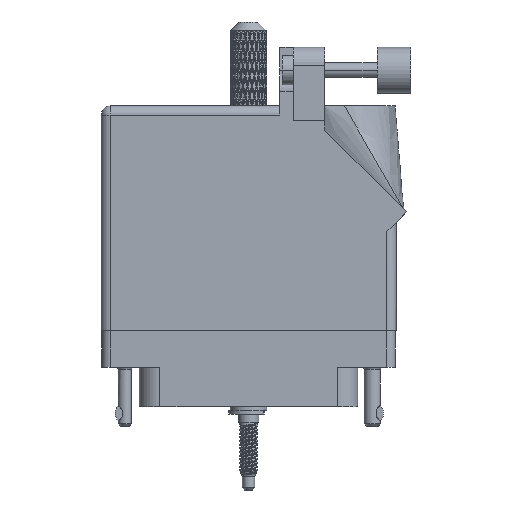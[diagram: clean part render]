
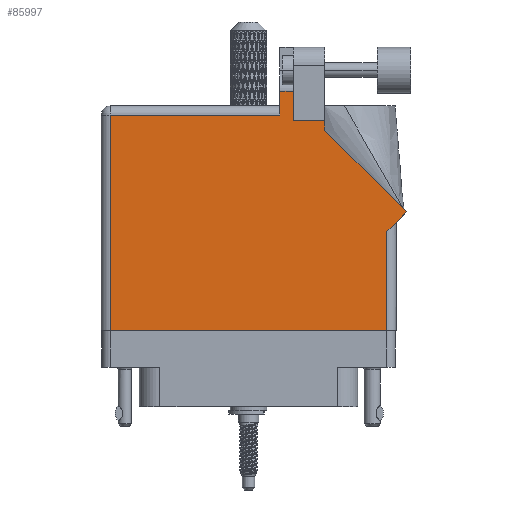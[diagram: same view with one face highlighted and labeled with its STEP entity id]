
A CAD part, front view. The second image highlights one B-rep face of the part: STEP entity #85997.
In plain terms, the highlighted face is planar.
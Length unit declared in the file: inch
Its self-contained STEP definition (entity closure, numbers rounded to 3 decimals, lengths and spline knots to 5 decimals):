
#2306 = VERTEX_POINT ( 'NONE', #101759 ) ;
#2897 = DIRECTION ( 'NONE',  ( 0., 1., 0. ) ) ;
#3239 = CARTESIAN_POINT ( 'NONE',  ( 0.212, 1.368, 0.455 ) ) ;
#4453 = DIRECTION ( 'NONE',  ( -1., 0., 0. ) ) ;
#6810 = DIRECTION ( 'NONE',  ( 0., 1., 0. ) ) ;
#7389 = VERTEX_POINT ( 'NONE', #38934 ) ;
#9613 = VERTEX_POINT ( 'NONE', #34563 ) ;
#9831 = DIRECTION ( 'NONE',  ( 0., -1., 0. ) ) ;
#12587 = ORIENTED_EDGE ( 'NONE', *, *, #70908, .T. ) ;
#12631 = VERTEX_POINT ( 'NONE', #112125 ) ;
#15644 = VECTOR ( 'NONE', #4453, 39.37008 ) ;
#15901 = CARTESIAN_POINT ( 'NONE',  ( 0.63677, 1.5315, 0.455 ) ) ;
#16752 = VECTOR ( 'NONE', #88255, 39.37008 ) ;
#16868 = FACE_OUTER_BOUND ( 'NONE', #62920, .T. ) ;
#25154 = LINE ( 'NONE', #15901, #16752 ) ;
#26247 = ORIENTED_EDGE ( 'NONE', *, *, #63996, .T. ) ;
#26473 = LINE ( 'NONE', #26677, #29269 ) ;
#26677 = CARTESIAN_POINT ( 'NONE',  ( 0.212, 1.43, 0.455 ) ) ;
#26872 = DIRECTION ( 'NONE',  ( -0.707, 0.707, 0. ) ) ;
#27418 = ORIENTED_EDGE ( 'NONE', *, *, #92689, .T. ) ;
#29269 = VECTOR ( 'NONE', #9831, 39.37008 ) ;
#30598 = ORIENTED_EDGE ( 'NONE', *, *, #83921, .T. ) ;
#31255 = ORIENTED_EDGE ( 'NONE', *, *, #103829, .T. ) ;
#32099 = CARTESIAN_POINT ( 'NONE',  ( -0.943, -0.1, 0.455 ) ) ;
#33418 = VERTEX_POINT ( 'NONE', #100658 ) ;
#34277 = CARTESIAN_POINT ( 'NONE',  ( -1.005, -0.1, 0.455 ) ) ;
#34563 = CARTESIAN_POINT ( 'NONE',  ( 0.212, 1.5315, 0.455 ) ) ;
#34659 = DIRECTION ( 'NONE',  ( 1., 0., 0. ) ) ;
#35789 = DIRECTION ( 'NONE',  ( 0., 0., -1. ) ) ;
#37146 = VECTOR ( 'NONE', #2897, 39.37008 ) ;
#38934 = CARTESIAN_POINT ( 'NONE',  ( 0.519, 1.33, 0.455 ) ) ;
#39125 = LINE ( 'NONE', #103367, #89053 ) ;
#39825 = CARTESIAN_POINT ( 'NONE',  ( 1.005, 0.637, 0.455 ) ) ;
#41065 = CARTESIAN_POINT ( 'NONE',  ( -1.005, 1.368, 0.455 ) ) ;
#43443 = CARTESIAN_POINT ( 'NONE',  ( 0.519, 1.26442, 0.455 ) ) ;
#43449 = VECTOR ( 'NONE', #89734, 39.37008 ) ;
#44180 = VECTOR ( 'NONE', #103181, 39.37008 ) ;
#44308 = PLANE ( 'NONE',  #67310 ) ;
#45299 = EDGE_CURVE ( 'NONE', #111157, #33418, #77032, .T. ) ;
#48701 = LINE ( 'NONE', #58874, #55599 ) ;
#52545 = VECTOR ( 'NONE', #111416, 39.37008 ) ;
#53640 = CARTESIAN_POINT ( 'NONE',  ( -1.005, 1.43, 0.455 ) ) ;
#55599 = VECTOR ( 'NONE', #59237, 39.37008 ) ;
#57001 = EDGE_CURVE ( 'NONE', #91630, #70174, #70779, .T. ) ;
#57333 = ORIENTED_EDGE ( 'NONE', *, *, #57001, .T. ) ;
#58874 = CARTESIAN_POINT ( 'NONE',  ( 0.519, 1.26442, 0.455 ) ) ;
#59237 = DIRECTION ( 'NONE',  ( 0., 1., 0. ) ) ;
#59428 = CARTESIAN_POINT ( 'NONE',  ( 0.306, 1.5315, 0.455 ) ) ;
#62920 = EDGE_LOOP ( 'NONE', ( #31255, #12587, #73707, #26247, #63160, #97047, #86370, #27418, #57333, #86699, #30598 ) ) ;
#63160 = ORIENTED_EDGE ( 'NONE', *, *, #91915, .T. ) ;
#63996 = EDGE_CURVE ( 'NONE', #86581, #2306, #103402, .T. ) ;
#66925 = EDGE_CURVE ( 'NONE', #70174, #7389, #48701, .T. ) ;
#67134 = LINE ( 'NONE', #114699, #43449 ) ;
#67310 = AXIS2_PLACEMENT_3D ( 'NONE', #53640, #35789, #114741 ) ;
#69325 = LINE ( 'NONE', #102088, #37146 ) ;
#70174 = VERTEX_POINT ( 'NONE', #43443 ) ;
#70779 = LINE ( 'NONE', #113625, #90266 ) ;
#70908 = EDGE_CURVE ( 'NONE', #93384, #9613, #25154, .T. ) ;
#73464 = LINE ( 'NONE', #39825, #44180 ) ;
#73707 = ORIENTED_EDGE ( 'NONE', *, *, #86479, .T. ) ;
#77032 = LINE ( 'NONE', #34277, #93613 ) ;
#83583 = VERTEX_POINT ( 'NONE', #89110 ) ;
#83921 = EDGE_CURVE ( 'NONE', #7389, #83583, #67134, .T. ) ;
#85997 = ADVANCED_FACE ( 'NONE', ( #16868 ), #44308, .F. ) ;
#86370 = ORIENTED_EDGE ( 'NONE', *, *, #92242, .T. ) ;
#86479 = EDGE_CURVE ( 'NONE', #9613, #86581, #26473, .T. ) ;
#86581 = VERTEX_POINT ( 'NONE', #3239 ) ;
#86699 = ORIENTED_EDGE ( 'NONE', *, *, #66925, .T. ) ;
#88255 = DIRECTION ( 'NONE',  ( -1., 0., 0. ) ) ;
#89053 = VECTOR ( 'NONE', #6810, 39.37008 ) ;
#89110 = CARTESIAN_POINT ( 'NONE',  ( 0.306, 1.33, 0.455 ) ) ;
#89734 = DIRECTION ( 'NONE',  ( -1., 0., 0. ) ) ;
#90266 = VECTOR ( 'NONE', #26872, 39.37008 ) ;
#90490 = CARTESIAN_POINT ( 'NONE',  ( -0.943, -0.1, 0.455 ) ) ;
#91630 = VERTEX_POINT ( 'NONE', #102996 ) ;
#91915 = EDGE_CURVE ( 'NONE', #2306, #111157, #99806, .T. ) ;
#92242 = EDGE_CURVE ( 'NONE', #33418, #12631, #69325, .T. ) ;
#92689 = EDGE_CURVE ( 'NONE', #12631, #91630, #73464, .T. ) ;
#93384 = VERTEX_POINT ( 'NONE', #59428 ) ;
#93613 = VECTOR ( 'NONE', #34659, 39.37008 ) ;
#97047 = ORIENTED_EDGE ( 'NONE', *, *, #45299, .T. ) ;
#99806 = LINE ( 'NONE', #32099, #52545 ) ;
#100658 = CARTESIAN_POINT ( 'NONE',  ( 0.943, -0.1, 0.455 ) ) ;
#101759 = CARTESIAN_POINT ( 'NONE',  ( -0.943, 1.368, 0.455 ) ) ;
#102088 = CARTESIAN_POINT ( 'NONE',  ( 0.943, 0.637, 0.455 ) ) ;
#102996 = CARTESIAN_POINT ( 'NONE',  ( 1.07571, 0.70771, 0.455 ) ) ;
#103181 = DIRECTION ( 'NONE',  ( 0.707, 0.707, 0. ) ) ;
#103367 = CARTESIAN_POINT ( 'NONE',  ( 0.306, 1.33, 0.455 ) ) ;
#103402 = LINE ( 'NONE', #41065, #15644 ) ;
#103829 = EDGE_CURVE ( 'NONE', #83583, #93384, #39125, .T. ) ;
#111157 = VERTEX_POINT ( 'NONE', #90490 ) ;
#111416 = DIRECTION ( 'NONE',  ( 0., -1., 0. ) ) ;
#112125 = CARTESIAN_POINT ( 'NONE',  ( 0.943, 0.575, 0.455 ) ) ;
#113625 = CARTESIAN_POINT ( 'NONE',  ( 1.07571, 0.70771, 0.455 ) ) ;
#114699 = CARTESIAN_POINT ( 'NONE',  ( 0.519, 1.33, 0.455 ) ) ;
#114741 = DIRECTION ( 'NONE',  ( -1., 0., 0. ) ) ;
